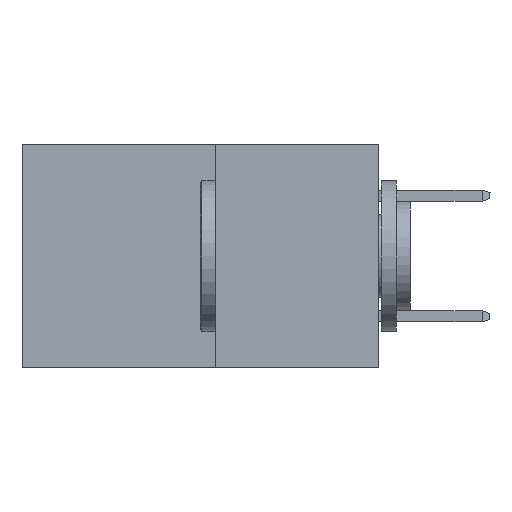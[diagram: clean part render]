
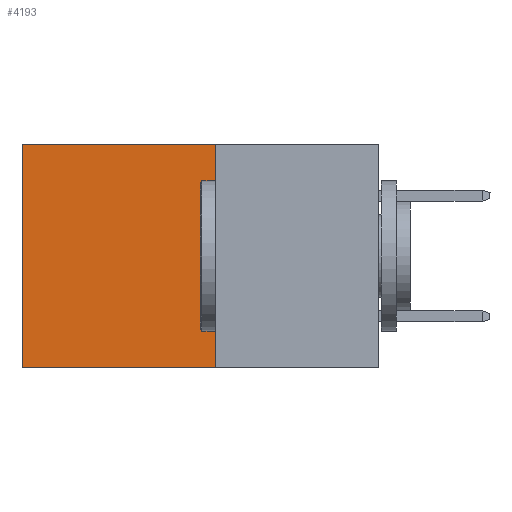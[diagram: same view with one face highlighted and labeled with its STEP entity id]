
A CAD part, left-side view. The second image highlights one B-rep face of the part: STEP entity #4193.
In plain terms, the highlighted planar face has unit normal (-1, 0, 0).
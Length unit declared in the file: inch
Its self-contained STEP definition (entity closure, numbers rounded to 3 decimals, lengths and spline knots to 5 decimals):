
#35 = FACE_OUTER_BOUND ( 'NONE', #8415, .T. ) ;
#661 = LINE ( 'NONE', #10384, #10747 ) ;
#1181 = DIRECTION ( 'NONE',  ( 0., 0., -1. ) ) ;
#2015 = LINE ( 'NONE', #4278, #2396 ) ;
#2123 = LINE ( 'NONE', #13532, #5909 ) ;
#2396 = VECTOR ( 'NONE', #11842, 39.37008 ) ;
#2675 = VERTEX_POINT ( 'NONE', #9943 ) ;
#2684 = DIRECTION ( 'NONE',  ( 1., 0., 0. ) ) ;
#2755 = EDGE_CURVE ( 'NONE', #3333, #6152, #661, .T. ) ;
#3333 = VERTEX_POINT ( 'NONE', #3449 ) ;
#3449 = CARTESIAN_POINT ( 'NONE',  ( 0.277, 0.27, 0. ) ) ;
#3890 = LINE ( 'NONE', #12330, #12812 ) ;
#4193 = ADVANCED_FACE ( 'NONE', ( #35 ), #14300, .F. ) ;
#4278 = CARTESIAN_POINT ( 'NONE',  ( 0.277, 0.59, -0.37 ) ) ;
#4761 = CARTESIAN_POINT ( 'NONE',  ( 0.277, 0.27, -0.37 ) ) ;
#5157 = ORIENTED_EDGE ( 'NONE', *, *, #7037, .F. ) ;
#5820 = AXIS2_PLACEMENT_3D ( 'NONE', #4761, #2684, #1181 ) ;
#5909 = VECTOR ( 'NONE', #13540, 39.37008 ) ;
#6152 = VERTEX_POINT ( 'NONE', #10983 ) ;
#7037 = EDGE_CURVE ( 'NONE', #6152, #9533, #2123, .T. ) ;
#7212 = EDGE_CURVE ( 'NONE', #3333, #2675, #3890, .T. ) ;
#8415 = EDGE_LOOP ( 'NONE', ( #10620, #5157, #12472, #10083 ) ) ;
#9533 = VERTEX_POINT ( 'NONE', #12480 ) ;
#9943 = CARTESIAN_POINT ( 'NONE',  ( 0.277, 0.59, 0. ) ) ;
#10083 = ORIENTED_EDGE ( 'NONE', *, *, #7212, .T. ) ;
#10384 = CARTESIAN_POINT ( 'NONE',  ( 0.277, 0.27, -0.37 ) ) ;
#10620 = ORIENTED_EDGE ( 'NONE', *, *, #15243, .T. ) ;
#10747 = VECTOR ( 'NONE', #11749, 39.37008 ) ;
#10983 = CARTESIAN_POINT ( 'NONE',  ( 0.277, 0.27, -0.37 ) ) ;
#11749 = DIRECTION ( 'NONE',  ( 0., 0., -1. ) ) ;
#11842 = DIRECTION ( 'NONE',  ( 0., 0., -1. ) ) ;
#12330 = CARTESIAN_POINT ( 'NONE',  ( 0.277, 0.27, 0. ) ) ;
#12382 = DIRECTION ( 'NONE',  ( 0., 1., 0. ) ) ;
#12472 = ORIENTED_EDGE ( 'NONE', *, *, #2755, .F. ) ;
#12480 = CARTESIAN_POINT ( 'NONE',  ( 0.277, 0.59, -0.37 ) ) ;
#12812 = VECTOR ( 'NONE', #12382, 39.37008 ) ;
#13532 = CARTESIAN_POINT ( 'NONE',  ( 0.277, 0.27, -0.37 ) ) ;
#13540 = DIRECTION ( 'NONE',  ( 0., 1., 0. ) ) ;
#14300 = PLANE ( 'NONE',  #5820 ) ;
#15243 = EDGE_CURVE ( 'NONE', #2675, #9533, #2015, .T. ) ;
